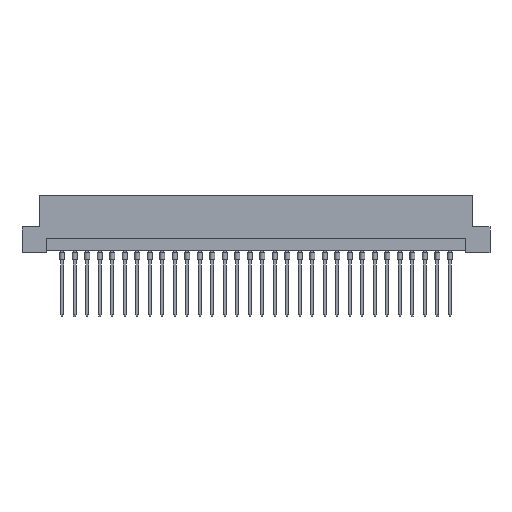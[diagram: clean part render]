
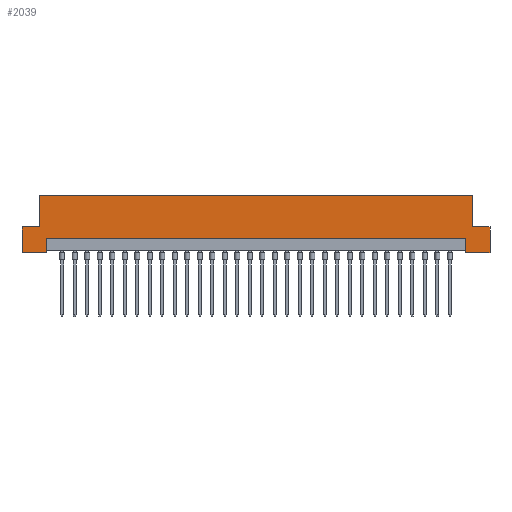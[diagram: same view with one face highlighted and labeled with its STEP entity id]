
A CAD part, front view. The second image highlights one B-rep face of the part: STEP entity #2039.
In plain terms, the highlighted planar face has unit normal (0, -1, 0).
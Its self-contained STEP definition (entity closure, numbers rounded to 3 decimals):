
#112 = LINE ( 'NONE', #5864, #7224 ) ;
#194 = VECTOR ( 'NONE', #16565, 1000. ) ;
#207 = VECTOR ( 'NONE', #16651, 1000. ) ;
#485 = DIRECTION ( 'NONE',  ( 0., 0., -1. ) ) ;
#491 = EDGE_LOOP ( 'NONE', ( #16968, #16123, #15263, #2082, #4452, #13772, #13100, #14654, #14393, #3361, #3797, #4158 ) ) ;
#529 = EDGE_CURVE ( 'NONE', #14298, #4157, #112, .T. ) ;
#676 = VECTOR ( 'NONE', #13345, 1000. ) ;
#859 = EDGE_CURVE ( 'NONE', #5163, #14298, #5387, .T. ) ;
#1346 = VERTEX_POINT ( 'NONE', #6101 ) ;
#1449 = EDGE_CURVE ( 'NONE', #12868, #5163, #18215, .T. ) ;
#1855 = EDGE_CURVE ( 'NONE', #15297, #9140, #4643, .T. ) ;
#2002 = CARTESIAN_POINT ( 'NONE',  ( -47.5, 0., 0. ) ) ;
#2011 = DIRECTION ( 'NONE',  ( -1., 0., 0. ) ) ;
#2039 = ADVANCED_FACE ( 'NONE', ( #5389 ), #17049, .F. ) ;
#2082 = ORIENTED_EDGE ( 'NONE', *, *, #4701, .F. ) ;
#2090 = EDGE_CURVE ( 'NONE', #9140, #12868, #6900, .T. ) ;
#2791 = LINE ( 'NONE', #15235, #5846 ) ;
#3353 = CARTESIAN_POINT ( 'NONE',  ( 47.5, 0., 0. ) ) ;
#3361 = ORIENTED_EDGE ( 'NONE', *, *, #1449, .F. ) ;
#3473 = CARTESIAN_POINT ( 'NONE',  ( 42.6, 0., 0. ) ) ;
#3797 = ORIENTED_EDGE ( 'NONE', *, *, #2090, .F. ) ;
#4157 = VERTEX_POINT ( 'NONE', #13141 ) ;
#4158 = ORIENTED_EDGE ( 'NONE', *, *, #1855, .F. ) ;
#4299 = VECTOR ( 'NONE', #9823, 1000. ) ;
#4303 = LINE ( 'NONE', #14146, #13383 ) ;
#4436 = EDGE_CURVE ( 'NONE', #4157, #5404, #2791, .T. ) ;
#4452 = ORIENTED_EDGE ( 'NONE', *, *, #9152, .F. ) ;
#4524 = VECTOR ( 'NONE', #9642, 1000. ) ;
#4643 = LINE ( 'NONE', #10404, #676 ) ;
#4701 = EDGE_CURVE ( 'NONE', #15074, #8533, #7697, .T. ) ;
#5163 = VERTEX_POINT ( 'NONE', #9280 ) ;
#5387 = LINE ( 'NONE', #18189, #4524 ) ;
#5389 = FACE_OUTER_BOUND ( 'NONE', #491, .T. ) ;
#5404 = VERTEX_POINT ( 'NONE', #11168 ) ;
#5846 = VECTOR ( 'NONE', #13811, 1000. ) ;
#5864 = CARTESIAN_POINT ( 'NONE',  ( -44., 0., 5.2 ) ) ;
#6101 = CARTESIAN_POINT ( 'NONE',  ( 44., 0., 5.2 ) ) ;
#6652 = VECTOR ( 'NONE', #7967, 1000. ) ;
#6900 = LINE ( 'NONE', #9644, #4299 ) ;
#6940 = DIRECTION ( 'NONE',  ( -1., 0., 0. ) ) ;
#6961 = CARTESIAN_POINT ( 'NONE',  ( 47.5, 0., 5.2 ) ) ;
#7224 = VECTOR ( 'NONE', #17425, 1000. ) ;
#7697 = LINE ( 'NONE', #3353, #13416 ) ;
#7791 = DIRECTION ( 'NONE',  ( 0., 0., -1. ) ) ;
#7967 = DIRECTION ( 'NONE',  ( 0., 0., 1. ) ) ;
#8533 = VERTEX_POINT ( 'NONE', #12114 ) ;
#8573 = CARTESIAN_POINT ( 'NONE',  ( -42.6, 0., 2.9 ) ) ;
#8887 = CARTESIAN_POINT ( 'NONE',  ( 42.6, 0., 2.9 ) ) ;
#9140 = VERTEX_POINT ( 'NONE', #10761 ) ;
#9152 = EDGE_CURVE ( 'NONE', #1346, #15074, #10663, .T. ) ;
#9280 = CARTESIAN_POINT ( 'NONE',  ( -47.5, 0., 5.2 ) ) ;
#9434 = CARTESIAN_POINT ( 'NONE',  ( 47.5, 0., 5.2 ) ) ;
#9642 = DIRECTION ( 'NONE',  ( 1., 0., 0. ) ) ;
#9644 = CARTESIAN_POINT ( 'NONE',  ( -47.5, 0., 0. ) ) ;
#9730 = AXIS2_PLACEMENT_3D ( 'NONE', #14183, #18462, #12673 ) ;
#9823 = DIRECTION ( 'NONE',  ( -1., 0., 0. ) ) ;
#9989 = EDGE_CURVE ( 'NONE', #8533, #13838, #13627, .T. ) ;
#10404 = CARTESIAN_POINT ( 'NONE',  ( -42.6, 0., 0.5 ) ) ;
#10463 = EDGE_CURVE ( 'NONE', #12729, #13838, #15039, .T. ) ;
#10663 = LINE ( 'NONE', #9434, #194 ) ;
#10761 = CARTESIAN_POINT ( 'NONE',  ( -42.6, 0., 0. ) ) ;
#10949 = CARTESIAN_POINT ( 'NONE',  ( 44., 0., 5.2 ) ) ;
#11168 = CARTESIAN_POINT ( 'NONE',  ( 44., 0., 11.6 ) ) ;
#11573 = CARTESIAN_POINT ( 'NONE',  ( -44., 0., 5.2 ) ) ;
#11803 = CARTESIAN_POINT ( 'NONE',  ( 42.6, 0., 0.5 ) ) ;
#12002 = VECTOR ( 'NONE', #485, 1000. ) ;
#12114 = CARTESIAN_POINT ( 'NONE',  ( 47.5, 0., 0. ) ) ;
#12673 = DIRECTION ( 'NONE',  ( 0., 0., 1. ) ) ;
#12729 = VERTEX_POINT ( 'NONE', #8887 ) ;
#12868 = VERTEX_POINT ( 'NONE', #2002 ) ;
#13100 = ORIENTED_EDGE ( 'NONE', *, *, #4436, .F. ) ;
#13141 = CARTESIAN_POINT ( 'NONE',  ( -44., 0., 11.6 ) ) ;
#13345 = DIRECTION ( 'NONE',  ( 0., 0., -1. ) ) ;
#13383 = VECTOR ( 'NONE', #6940, 1000. ) ;
#13416 = VECTOR ( 'NONE', #7791, 1000. ) ;
#13627 = LINE ( 'NONE', #16215, #14127 ) ;
#13772 = ORIENTED_EDGE ( 'NONE', *, *, #15083, .T. ) ;
#13811 = DIRECTION ( 'NONE',  ( 1., 0., 0. ) ) ;
#13838 = VERTEX_POINT ( 'NONE', #3473 ) ;
#14127 = VECTOR ( 'NONE', #2011, 1000. ) ;
#14146 = CARTESIAN_POINT ( 'NONE',  ( 42.6, 0., 2.9 ) ) ;
#14183 = CARTESIAN_POINT ( 'NONE',  ( -47.5, 0., 11.6 ) ) ;
#14298 = VERTEX_POINT ( 'NONE', #11573 ) ;
#14393 = ORIENTED_EDGE ( 'NONE', *, *, #859, .F. ) ;
#14654 = ORIENTED_EDGE ( 'NONE', *, *, #529, .F. ) ;
#15039 = LINE ( 'NONE', #11803, #12002 ) ;
#15074 = VERTEX_POINT ( 'NONE', #6961 ) ;
#15083 = EDGE_CURVE ( 'NONE', #1346, #5404, #18276, .T. ) ;
#15235 = CARTESIAN_POINT ( 'NONE',  ( -47.5, 0., 11.6 ) ) ;
#15263 = ORIENTED_EDGE ( 'NONE', *, *, #9989, .F. ) ;
#15297 = VERTEX_POINT ( 'NONE', #8573 ) ;
#15706 = EDGE_CURVE ( 'NONE', #12729, #15297, #4303, .T. ) ;
#16123 = ORIENTED_EDGE ( 'NONE', *, *, #10463, .T. ) ;
#16215 = CARTESIAN_POINT ( 'NONE',  ( -47.5, 0., 0. ) ) ;
#16565 = DIRECTION ( 'NONE',  ( 1., 0., 0. ) ) ;
#16651 = DIRECTION ( 'NONE',  ( 0., 0., 1. ) ) ;
#16968 = ORIENTED_EDGE ( 'NONE', *, *, #15706, .F. ) ;
#17049 = PLANE ( 'NONE',  #9730 ) ;
#17425 = DIRECTION ( 'NONE',  ( 0., 0., 1. ) ) ;
#18121 = CARTESIAN_POINT ( 'NONE',  ( -47.5, 0., 0. ) ) ;
#18189 = CARTESIAN_POINT ( 'NONE',  ( -47.5, 0., 5.2 ) ) ;
#18215 = LINE ( 'NONE', #18121, #6652 ) ;
#18276 = LINE ( 'NONE', #10949, #207 ) ;
#18462 = DIRECTION ( 'NONE',  ( 0., 1., 0. ) ) ;
